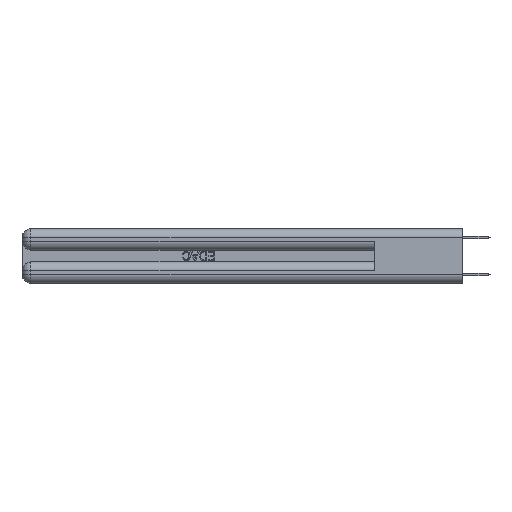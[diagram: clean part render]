
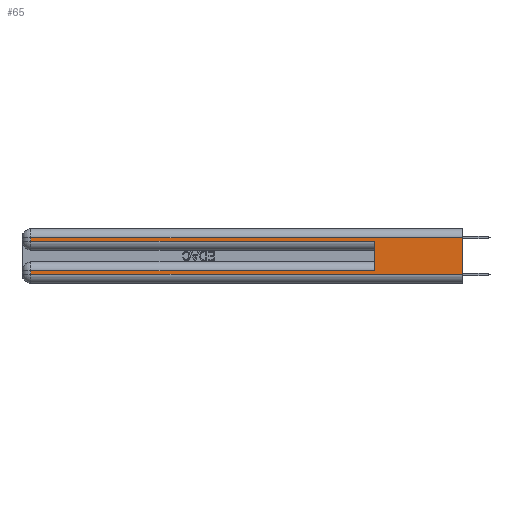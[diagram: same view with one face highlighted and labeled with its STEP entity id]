
A CAD part, left-side view. The second image highlights one B-rep face of the part: STEP entity #65.
In plain terms, the highlighted planar face has unit normal (-1, 0, 0).
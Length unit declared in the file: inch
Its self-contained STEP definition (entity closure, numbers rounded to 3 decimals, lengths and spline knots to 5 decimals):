
#65 = ADVANCED_FACE ( 'NONE', ( #13754 ), #6271, .F. ) ;
#209 = LINE ( 'NONE', #20458, #10788 ) ;
#805 = CARTESIAN_POINT ( 'NONE',  ( 0., 0.6, 0.145 ) ) ;
#1208 = CARTESIAN_POINT ( 'NONE',  ( 0., 2.94, 0.06 ) ) ;
#1715 = CARTESIAN_POINT ( 'NONE',  ( 0., 0.6, 0.085 ) ) ;
#2317 = VECTOR ( 'NONE', #30216, 39.37008 ) ;
#2768 = DIRECTION ( 'NONE',  ( 0., 0., -1. ) ) ;
#2791 = EDGE_CURVE ( 'NONE', #24888, #10962, #8014, .T. ) ;
#3152 = VECTOR ( 'NONE', #20069, 39.37008 ) ;
#3347 = LINE ( 'NONE', #11832, #16012 ) ;
#3499 = ORIENTED_EDGE ( 'NONE', *, *, #17770, .T. ) ;
#3976 = EDGE_CURVE ( 'NONE', #10962, #9958, #209, .T. ) ;
#6271 = PLANE ( 'NONE',  #25261 ) ;
#7425 = CARTESIAN_POINT ( 'NONE',  ( 0., 0., 0.06 ) ) ;
#8014 = LINE ( 'NONE', #26093, #12920 ) ;
#8184 = EDGE_CURVE ( 'NONE', #26212, #32605, #31355, .T. ) ;
#8259 = CARTESIAN_POINT ( 'NONE',  ( 0., 2.94, 0.285 ) ) ;
#8771 = DIRECTION ( 'NONE',  ( 0., -1., 0. ) ) ;
#9958 = VERTEX_POINT ( 'NONE', #7425 ) ;
#10471 = LINE ( 'NONE', #20707, #28502 ) ;
#10562 = DIRECTION ( 'NONE',  ( 0., -1., 0. ) ) ;
#10788 = VECTOR ( 'NONE', #10562, 39.37008 ) ;
#10915 = EDGE_LOOP ( 'NONE', ( #30424, #24042, #16610, #17122, #26238, #3499, #15656, #12394 ) ) ;
#10962 = VERTEX_POINT ( 'NONE', #1208 ) ;
#11621 = EDGE_CURVE ( 'NONE', #21857, #22351, #10471, .T. ) ;
#11832 = CARTESIAN_POINT ( 'NONE',  ( 0., 0., 0.285 ) ) ;
#12065 = LINE ( 'NONE', #14265, #31491 ) ;
#12271 = LINE ( 'NONE', #25228, #2317 ) ;
#12394 = ORIENTED_EDGE ( 'NONE', *, *, #3976, .T. ) ;
#12864 = EDGE_CURVE ( 'NONE', #29488, #32605, #3347, .T. ) ;
#12920 = VECTOR ( 'NONE', #2768, 39.37008 ) ;
#13754 = FACE_OUTER_BOUND ( 'NONE', #10915, .T. ) ;
#14265 = CARTESIAN_POINT ( 'NONE',  ( 0., 2.94, 0.37 ) ) ;
#15588 = DIRECTION ( 'NONE',  ( 0., 1., 0. ) ) ;
#15656 = ORIENTED_EDGE ( 'NONE', *, *, #2791, .T. ) ;
#16012 = VECTOR ( 'NONE', #8771, 39.37008 ) ;
#16610 = ORIENTED_EDGE ( 'NONE', *, *, #17624, .T. ) ;
#16821 = DIRECTION ( 'NONE',  ( 0., 0., -1. ) ) ;
#17122 = ORIENTED_EDGE ( 'NONE', *, *, #12864, .T. ) ;
#17624 = EDGE_CURVE ( 'NONE', #22351, #29488, #12065, .T. ) ;
#17770 = EDGE_CURVE ( 'NONE', #26212, #24888, #27941, .T. ) ;
#18691 = CARTESIAN_POINT ( 'NONE',  ( 0., 0., 0.37 ) ) ;
#18854 = DIRECTION ( 'NONE',  ( 1., 0., 0. ) ) ;
#20069 = DIRECTION ( 'NONE',  ( 0., 1., 0. ) ) ;
#20458 = CARTESIAN_POINT ( 'NONE',  ( 0., 0., 0.06 ) ) ;
#20707 = CARTESIAN_POINT ( 'NONE',  ( 0., 0., 0.31 ) ) ;
#21857 = VERTEX_POINT ( 'NONE', #21866 ) ;
#21866 = CARTESIAN_POINT ( 'NONE',  ( 0., 0., 0.31 ) ) ;
#22351 = VERTEX_POINT ( 'NONE', #24916 ) ;
#22631 = CARTESIAN_POINT ( 'NONE',  ( 0., 0., 0.085 ) ) ;
#24042 = ORIENTED_EDGE ( 'NONE', *, *, #11621, .T. ) ;
#24888 = VERTEX_POINT ( 'NONE', #30131 ) ;
#24916 = CARTESIAN_POINT ( 'NONE',  ( 0., 2.94, 0.31 ) ) ;
#25228 = CARTESIAN_POINT ( 'NONE',  ( 0., 0., 0.37 ) ) ;
#25261 = AXIS2_PLACEMENT_3D ( 'NONE', #18691, #18854, #16821 ) ;
#26093 = CARTESIAN_POINT ( 'NONE',  ( 0., 2.94, 0.37 ) ) ;
#26212 = VERTEX_POINT ( 'NONE', #1715 ) ;
#26238 = ORIENTED_EDGE ( 'NONE', *, *, #8184, .F. ) ;
#27941 = LINE ( 'NONE', #22631, #3152 ) ;
#28062 = CARTESIAN_POINT ( 'NONE',  ( 0., 0.6, 0.285 ) ) ;
#28502 = VECTOR ( 'NONE', #15588, 39.37008 ) ;
#29449 = DIRECTION ( 'NONE',  ( 0., 0., 1. ) ) ;
#29488 = VERTEX_POINT ( 'NONE', #8259 ) ;
#29667 = DIRECTION ( 'NONE',  ( 0., 0., -1. ) ) ;
#30131 = CARTESIAN_POINT ( 'NONE',  ( 0., 2.94, 0.085 ) ) ;
#30216 = DIRECTION ( 'NONE',  ( 0., 0., -1. ) ) ;
#30424 = ORIENTED_EDGE ( 'NONE', *, *, #33459, .F. ) ;
#31355 = LINE ( 'NONE', #805, #32608 ) ;
#31491 = VECTOR ( 'NONE', #29667, 39.37008 ) ;
#32605 = VERTEX_POINT ( 'NONE', #28062 ) ;
#32608 = VECTOR ( 'NONE', #29449, 39.37008 ) ;
#33459 = EDGE_CURVE ( 'NONE', #21857, #9958, #12271, .T. ) ;
